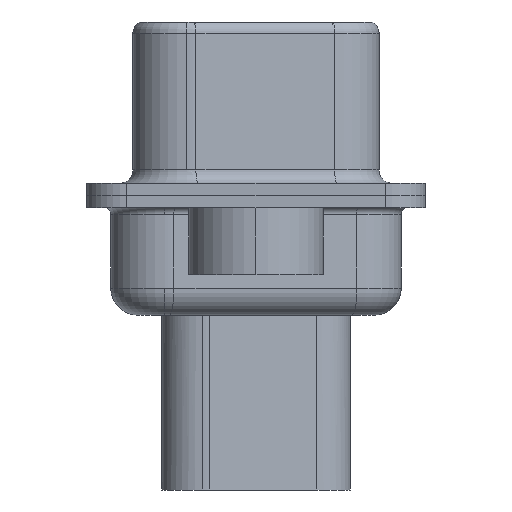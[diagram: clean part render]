
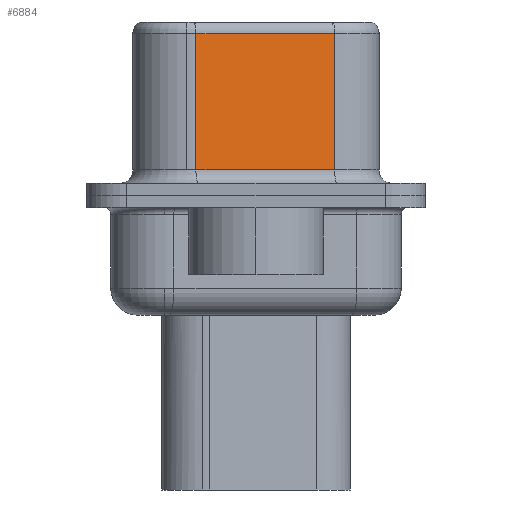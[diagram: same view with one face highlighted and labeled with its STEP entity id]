
A CAD part, left-side view. The second image highlights one B-rep face of the part: STEP entity #6884.
In plain terms, the highlighted planar face has unit normal (-0.985, -0.174, 0).
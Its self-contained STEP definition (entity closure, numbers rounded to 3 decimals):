
#225 = EDGE_CURVE ( 'NONE', #9521, #10372, #10592, .T. ) ;
#1649 = DIRECTION ( 'NONE',  ( -0.174, 0.985, 0. ) ) ;
#2114 = VERTEX_POINT ( 'NONE', #7809 ) ;
#3743 = ORIENTED_EDGE ( 'NONE', *, *, #17913, .T. ) ;
#3926 = ORIENTED_EDGE ( 'NONE', *, *, #17436, .T. ) ;
#4529 = CARTESIAN_POINT ( 'NONE',  ( 3.67, 2.233, 6.02 ) ) ;
#4597 = EDGE_LOOP ( 'NONE', ( #17519, #3743, #3926, #14665 ) ) ;
#4753 = CARTESIAN_POINT ( 'NONE',  ( 3.67, 2.233, 0.95 ) ) ;
#5465 = DIRECTION ( 'NONE',  ( 0., 0., -1. ) ) ;
#5512 = AXIS2_PLACEMENT_3D ( 'NONE', #15200, #11401, #22012 ) ;
#5531 = VECTOR ( 'NONE', #1649, 1000. ) ;
#6489 = FACE_OUTER_BOUND ( 'NONE', #4597, .T. ) ;
#6884 = ADVANCED_FACE ( 'NONE', ( #6489 ), #16655, .F. ) ;
#7094 = EDGE_CURVE ( 'NONE', #2114, #10372, #10508, .T. ) ;
#7809 = CARTESIAN_POINT ( 'NONE',  ( 4.58, -2.927, 6.02 ) ) ;
#8906 = DIRECTION ( 'NONE',  ( 0.174, -0.985, 0. ) ) ;
#9521 = VERTEX_POINT ( 'NONE', #4753 ) ;
#10163 = LINE ( 'NONE', #16966, #5531 ) ;
#10372 = VERTEX_POINT ( 'NONE', #19246 ) ;
#10508 = LINE ( 'NONE', #17314, #19426 ) ;
#10592 = LINE ( 'NONE', #17176, #12806 ) ;
#11401 = DIRECTION ( 'NONE',  ( 0.985, 0.174, 0. ) ) ;
#11973 = CARTESIAN_POINT ( 'NONE',  ( 3.67, 2.233, 6.52 ) ) ;
#12505 = VERTEX_POINT ( 'NONE', #4529 ) ;
#12806 = VECTOR ( 'NONE', #8906, 1000. ) ;
#14665 = ORIENTED_EDGE ( 'NONE', *, *, #225, .T. ) ;
#15200 = CARTESIAN_POINT ( 'NONE',  ( 4.58, -2.927, 6.52 ) ) ;
#16655 = PLANE ( 'NONE',  #5512 ) ;
#16883 = LINE ( 'NONE', #11973, #17655 ) ;
#16966 = CARTESIAN_POINT ( 'NONE',  ( 4.58, -2.927, 6.02 ) ) ;
#17176 = CARTESIAN_POINT ( 'NONE',  ( 4.58, -2.927, 0.95 ) ) ;
#17314 = CARTESIAN_POINT ( 'NONE',  ( 4.58, -2.927, 6.52 ) ) ;
#17436 = EDGE_CURVE ( 'NONE', #12505, #9521, #16883, .T. ) ;
#17519 = ORIENTED_EDGE ( 'NONE', *, *, #7094, .F. ) ;
#17655 = VECTOR ( 'NONE', #18780, 1000. ) ;
#17913 = EDGE_CURVE ( 'NONE', #2114, #12505, #10163, .T. ) ;
#18780 = DIRECTION ( 'NONE',  ( 0., 0., -1. ) ) ;
#19246 = CARTESIAN_POINT ( 'NONE',  ( 4.58, -2.927, 0.95 ) ) ;
#19426 = VECTOR ( 'NONE', #5465, 1000. ) ;
#22012 = DIRECTION ( 'NONE',  ( -0.174, 0.985, 0. ) ) ;
